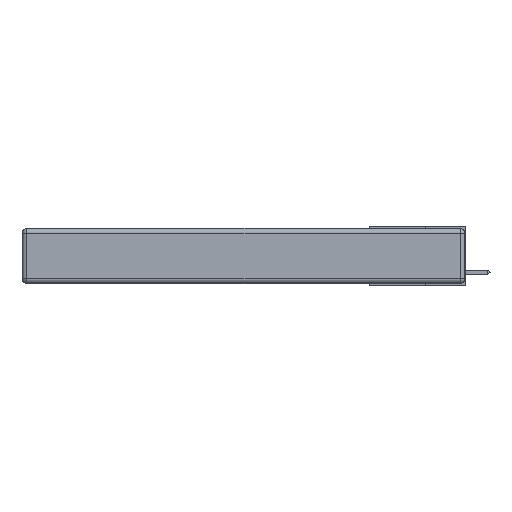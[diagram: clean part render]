
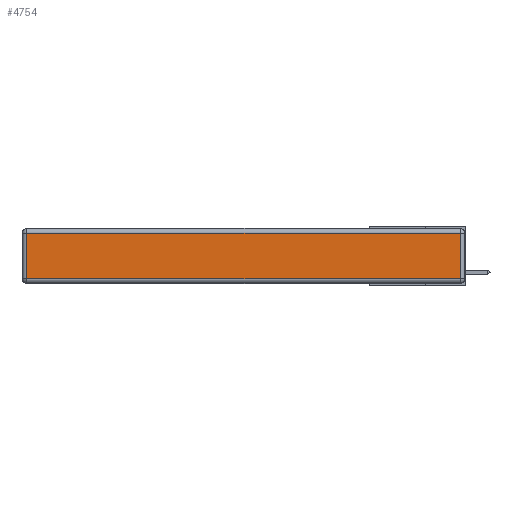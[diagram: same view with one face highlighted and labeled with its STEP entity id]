
A CAD part, left-side view. The second image highlights one B-rep face of the part: STEP entity #4754.
In plain terms, the highlighted planar face has unit normal (-1, 0, 0).
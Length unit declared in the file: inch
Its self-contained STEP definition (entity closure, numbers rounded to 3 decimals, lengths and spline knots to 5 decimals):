
#96 = VERTEX_POINT ( 'NONE', #12089 ) ;
#600 = LINE ( 'NONE', #8710, #20248 ) ;
#1843 = DIRECTION ( 'NONE',  ( 0., 0., 1. ) ) ;
#2751 = DIRECTION ( 'NONE',  ( 0., 0., 1. ) ) ;
#3338 = VERTEX_POINT ( 'NONE', #15687 ) ;
#4074 = CARTESIAN_POINT ( 'NONE',  ( 0., 0., -0.313 ) ) ;
#4505 = VECTOR ( 'NONE', #11256, 39.37008 ) ;
#4754 = ADVANCED_FACE ( 'NONE', ( #9623 ), #9125, .T. ) ;
#5072 = AXIS2_PLACEMENT_3D ( 'NONE', #16102, #16204, #2751 ) ;
#5432 = EDGE_CURVE ( 'NONE', #19035, #12642, #9913, .T. ) ;
#5931 = LINE ( 'NONE', #9389, #4505 ) ;
#6043 = DIRECTION ( 'NONE',  ( 0., -1., 0. ) ) ;
#6572 = VECTOR ( 'NONE', #6043, 39.37008 ) ;
#7459 = ORIENTED_EDGE ( 'NONE', *, *, #10322, .T. ) ;
#8710 = CARTESIAN_POINT ( 'NONE',  ( 0., 0.03, -0.343 ) ) ;
#9125 = PLANE ( 'NONE',  #5072 ) ;
#9389 = CARTESIAN_POINT ( 'NONE',  ( 0., 2.72, -0.343 ) ) ;
#9623 = FACE_OUTER_BOUND ( 'NONE', #19269, .T. ) ;
#9859 = EDGE_CURVE ( 'NONE', #12642, #3338, #5931, .T. ) ;
#9913 = LINE ( 'NONE', #20440, #15185 ) ;
#10322 = EDGE_CURVE ( 'NONE', #3338, #96, #17823, .T. ) ;
#10501 = ORIENTED_EDGE ( 'NONE', *, *, #5432, .T. ) ;
#11256 = DIRECTION ( 'NONE',  ( 0., 0., -1. ) ) ;
#12089 = CARTESIAN_POINT ( 'NONE',  ( 0., 0.03, -0.313 ) ) ;
#12642 = VERTEX_POINT ( 'NONE', #25188 ) ;
#15185 = VECTOR ( 'NONE', #25062, 39.37008 ) ;
#15687 = CARTESIAN_POINT ( 'NONE',  ( 0., 2.72, -0.313 ) ) ;
#16102 = CARTESIAN_POINT ( 'NONE',  ( 0., 0., -0.343 ) ) ;
#16204 = DIRECTION ( 'NONE',  ( -1., 0., 0. ) ) ;
#17001 = EDGE_CURVE ( 'NONE', #96, #19035, #600, .T. ) ;
#17823 = LINE ( 'NONE', #4074, #6572 ) ;
#19035 = VERTEX_POINT ( 'NONE', #28153 ) ;
#19269 = EDGE_LOOP ( 'NONE', ( #7459, #25148, #10501, #24628 ) ) ;
#20248 = VECTOR ( 'NONE', #1843, 39.37008 ) ;
#20440 = CARTESIAN_POINT ( 'NONE',  ( 0., 2.75, -0.03 ) ) ;
#24628 = ORIENTED_EDGE ( 'NONE', *, *, #9859, .T. ) ;
#25062 = DIRECTION ( 'NONE',  ( 0., 1., 0. ) ) ;
#25148 = ORIENTED_EDGE ( 'NONE', *, *, #17001, .T. ) ;
#25188 = CARTESIAN_POINT ( 'NONE',  ( 0., 2.72, -0.03 ) ) ;
#28153 = CARTESIAN_POINT ( 'NONE',  ( 0., 0.03, -0.03 ) ) ;
